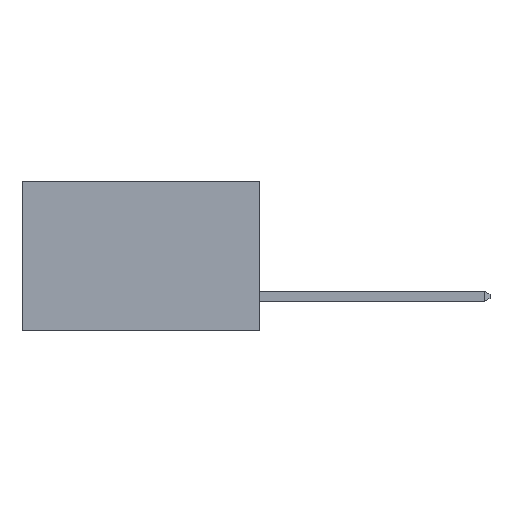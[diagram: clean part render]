
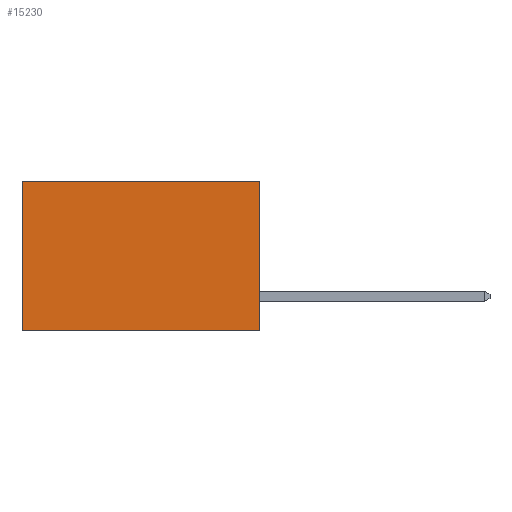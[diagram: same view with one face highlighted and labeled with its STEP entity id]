
A CAD part, left-side view. The second image highlights one B-rep face of the part: STEP entity #15230.
In plain terms, the highlighted planar face has unit normal (-1, 0, 0).
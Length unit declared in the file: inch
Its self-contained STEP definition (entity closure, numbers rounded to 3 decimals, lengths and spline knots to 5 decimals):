
#3 = VERTEX_POINT ( 'NONE', #2014 ) ;
#202 = VERTEX_POINT ( 'NONE', #4209 ) ;
#608 = CARTESIAN_POINT ( 'NONE',  ( 0.277, 0., -0.37 ) ) ;
#969 = EDGE_CURVE ( 'NONE', #202, #22461, #7386, .T. ) ;
#1700 = EDGE_CURVE ( 'NONE', #14425, #22461, #14636, .T. ) ;
#2014 = CARTESIAN_POINT ( 'NONE',  ( 0.277, 0., 0. ) ) ;
#2721 = CARTESIAN_POINT ( 'NONE',  ( 0.277, 0., -0.37 ) ) ;
#3997 = CARTESIAN_POINT ( 'NONE',  ( 0.277, 0., -0.37 ) ) ;
#4094 = ORIENTED_EDGE ( 'NONE', *, *, #16848, .T. ) ;
#4209 = CARTESIAN_POINT ( 'NONE',  ( 0.277, 0.59, 0. ) ) ;
#4667 = FACE_OUTER_BOUND ( 'NONE', #19458, .T. ) ;
#4740 = PLANE ( 'NONE',  #6356 ) ;
#5972 = DIRECTION ( 'NONE',  ( 0., 1., 0. ) ) ;
#6356 = AXIS2_PLACEMENT_3D ( 'NONE', #2721, #6744, #20752 ) ;
#6744 = DIRECTION ( 'NONE',  ( 1., 0., 0. ) ) ;
#7386 = LINE ( 'NONE', #17854, #12171 ) ;
#8040 = LINE ( 'NONE', #18013, #23901 ) ;
#8100 = DIRECTION ( 'NONE',  ( 0., 0., -1. ) ) ;
#8104 = ORIENTED_EDGE ( 'NONE', *, *, #1700, .F. ) ;
#8855 = CARTESIAN_POINT ( 'NONE',  ( 0.277, 0.59, -0.37 ) ) ;
#9647 = ORIENTED_EDGE ( 'NONE', *, *, #969, .T. ) ;
#9668 = LINE ( 'NONE', #3997, #14403 ) ;
#10506 = ORIENTED_EDGE ( 'NONE', *, *, #25299, .F. ) ;
#10896 = CARTESIAN_POINT ( 'NONE',  ( 0.277, 0., -0.37 ) ) ;
#12171 = VECTOR ( 'NONE', #8100, 39.37008 ) ;
#14403 = VECTOR ( 'NONE', #22009, 39.37008 ) ;
#14425 = VERTEX_POINT ( 'NONE', #10896 ) ;
#14636 = LINE ( 'NONE', #608, #24466 ) ;
#15230 = ADVANCED_FACE ( 'NONE', ( #4667 ), #4740, .F. ) ;
#16848 = EDGE_CURVE ( 'NONE', #3, #202, #8040, .T. ) ;
#17854 = CARTESIAN_POINT ( 'NONE',  ( 0.277, 0.59, -0.37 ) ) ;
#18013 = CARTESIAN_POINT ( 'NONE',  ( 0.277, 0., 0. ) ) ;
#19458 = EDGE_LOOP ( 'NONE', ( #9647, #8104, #10506, #4094 ) ) ;
#20245 = DIRECTION ( 'NONE',  ( 0., 1., 0. ) ) ;
#20752 = DIRECTION ( 'NONE',  ( 0., 0., -1. ) ) ;
#22009 = DIRECTION ( 'NONE',  ( 0., 0., -1. ) ) ;
#22461 = VERTEX_POINT ( 'NONE', #8855 ) ;
#23901 = VECTOR ( 'NONE', #5972, 39.37008 ) ;
#24466 = VECTOR ( 'NONE', #20245, 39.37008 ) ;
#25299 = EDGE_CURVE ( 'NONE', #3, #14425, #9668, .T. ) ;
